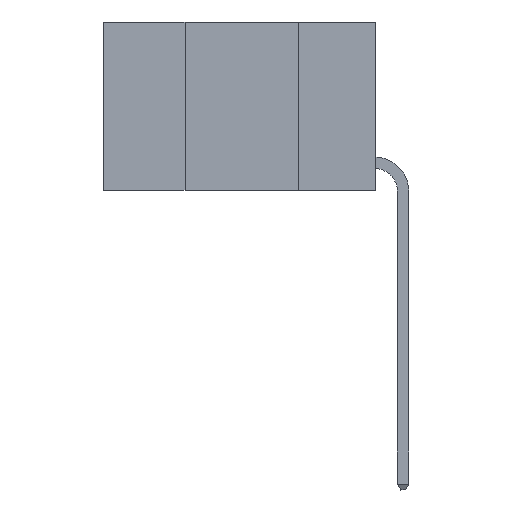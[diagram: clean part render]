
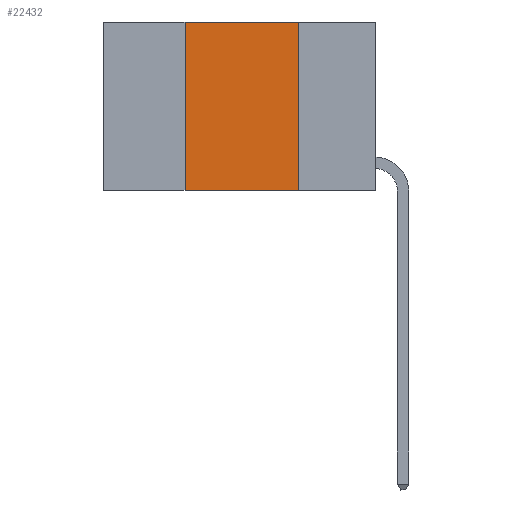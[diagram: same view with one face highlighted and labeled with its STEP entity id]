
A CAD part, left-side view. The second image highlights one B-rep face of the part: STEP entity #22432.
In plain terms, the highlighted planar face has unit normal (-1, 0, 0).
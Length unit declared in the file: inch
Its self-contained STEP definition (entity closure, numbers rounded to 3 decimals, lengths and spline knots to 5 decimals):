
#1044 = LINE ( 'NONE', #9286, #26644 ) ;
#1883 = CARTESIAN_POINT ( 'NONE',  ( 0., 0.42, -0.37 ) ) ;
#2995 = EDGE_CURVE ( 'NONE', #4132, #10739, #8974, .T. ) ;
#4132 = VERTEX_POINT ( 'NONE', #1883 ) ;
#5773 = CARTESIAN_POINT ( 'NONE',  ( 0., 0.17, -0.37 ) ) ;
#5866 = DIRECTION ( 'NONE',  ( 1., 0., 0. ) ) ;
#6386 = VECTOR ( 'NONE', #21445, 39.37008 ) ;
#8845 = VERTEX_POINT ( 'NONE', #11994 ) ;
#8974 = LINE ( 'NONE', #23353, #6386 ) ;
#9286 = CARTESIAN_POINT ( 'NONE',  ( 0., 0.6, 0. ) ) ;
#9376 = VECTOR ( 'NONE', #13868, 39.37008 ) ;
#9931 = FACE_OUTER_BOUND ( 'NONE', #25682, .T. ) ;
#10739 = VERTEX_POINT ( 'NONE', #24348 ) ;
#10857 = ORIENTED_EDGE ( 'NONE', *, *, #17449, .T. ) ;
#11607 = DIRECTION ( 'NONE',  ( 0., -1., 0. ) ) ;
#11851 = PLANE ( 'NONE',  #16016 ) ;
#11994 = CARTESIAN_POINT ( 'NONE',  ( 0., 0.17, 0. ) ) ;
#12109 = VERTEX_POINT ( 'NONE', #5773 ) ;
#13868 = DIRECTION ( 'NONE',  ( 0., -1., 0. ) ) ;
#14215 = ORIENTED_EDGE ( 'NONE', *, *, #24444, .F. ) ;
#15223 = VECTOR ( 'NONE', #26246, 39.37008 ) ;
#15506 = EDGE_CURVE ( 'NONE', #10739, #8845, #1044, .T. ) ;
#16016 = AXIS2_PLACEMENT_3D ( 'NONE', #22283, #5866, #24031 ) ;
#16314 = LINE ( 'NONE', #22040, #15223 ) ;
#17401 = ORIENTED_EDGE ( 'NONE', *, *, #2995, .F. ) ;
#17449 = EDGE_CURVE ( 'NONE', #4132, #12109, #20617, .T. ) ;
#19101 = ORIENTED_EDGE ( 'NONE', *, *, #15506, .F. ) ;
#20617 = LINE ( 'NONE', #24166, #9376 ) ;
#21445 = DIRECTION ( 'NONE',  ( 0., 0., 1. ) ) ;
#22040 = CARTESIAN_POINT ( 'NONE',  ( 0., 0.17, 0. ) ) ;
#22283 = CARTESIAN_POINT ( 'NONE',  ( 0., 0.6, 0. ) ) ;
#22432 = ADVANCED_FACE ( 'NONE', ( #9931 ), #11851, .F. ) ;
#23353 = CARTESIAN_POINT ( 'NONE',  ( 0., 0.42, 0. ) ) ;
#24031 = DIRECTION ( 'NONE',  ( 0., 0., -1. ) ) ;
#24166 = CARTESIAN_POINT ( 'NONE',  ( 0., 0.6, -0.37 ) ) ;
#24348 = CARTESIAN_POINT ( 'NONE',  ( 0., 0.42, 0. ) ) ;
#24444 = EDGE_CURVE ( 'NONE', #8845, #12109, #16314, .T. ) ;
#25682 = EDGE_LOOP ( 'NONE', ( #14215, #19101, #17401, #10857 ) ) ;
#26246 = DIRECTION ( 'NONE',  ( 0., 0., -1. ) ) ;
#26644 = VECTOR ( 'NONE', #11607, 39.37008 ) ;
